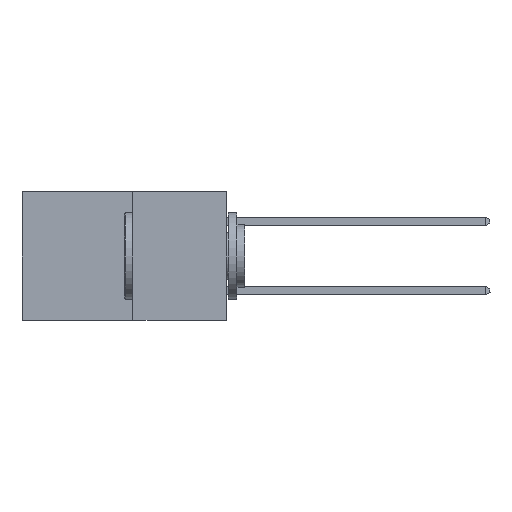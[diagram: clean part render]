
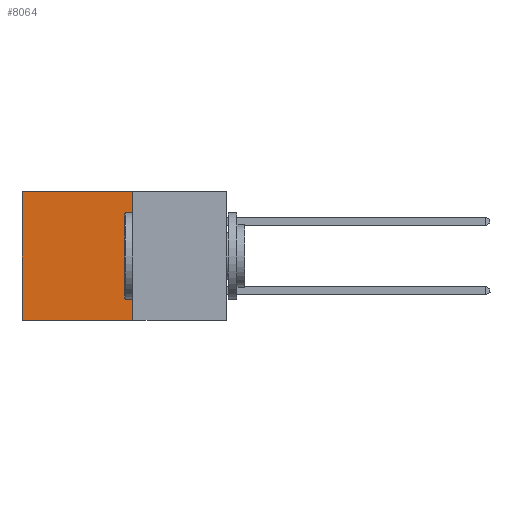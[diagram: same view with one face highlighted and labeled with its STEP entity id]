
A CAD part, left-side view. The second image highlights one B-rep face of the part: STEP entity #8064.
In plain terms, the highlighted planar face has unit normal (-1, 0, 0).
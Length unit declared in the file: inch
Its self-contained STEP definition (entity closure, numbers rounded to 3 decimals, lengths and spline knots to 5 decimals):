
#3552 = EDGE_CURVE ( 'NONE', #7562, #12265, #13279, .T. ) ;
#3914 = EDGE_CURVE ( 'NONE', #12431, #4497, #6377, .T. ) ;
#4263 = ORIENTED_EDGE ( 'NONE', *, *, #6254, .T. ) ;
#4317 = LINE ( 'NONE', #12335, #21337 ) ;
#4497 = VERTEX_POINT ( 'NONE', #16851 ) ;
#4714 = ORIENTED_EDGE ( 'NONE', *, *, #3552, .T. ) ;
#5039 = CARTESIAN_POINT ( 'NONE',  ( 0.277, 0.27, 0. ) ) ;
#5916 = LINE ( 'NONE', #16080, #13849 ) ;
#5930 = DIRECTION ( 'NONE',  ( 0., 0., -1. ) ) ;
#5969 = CARTESIAN_POINT ( 'NONE',  ( 0.277, 0.27, 0. ) ) ;
#6254 = EDGE_CURVE ( 'NONE', #12265, #4497, #4317, .T. ) ;
#6377 = LINE ( 'NONE', #14659, #6909 ) ;
#6710 = ORIENTED_EDGE ( 'NONE', *, *, #15152, .F. ) ;
#6909 = VECTOR ( 'NONE', #14686, 39.37008 ) ;
#7562 = VERTEX_POINT ( 'NONE', #5969 ) ;
#8064 = ADVANCED_FACE ( 'NONE', ( #17251 ), #18720, .F. ) ;
#9118 = EDGE_LOOP ( 'NONE', ( #4263, #14169, #6710, #4714 ) ) ;
#9193 = AXIS2_PLACEMENT_3D ( 'NONE', #18670, #18639, #18614 ) ;
#9762 = DIRECTION ( 'NONE',  ( 0., 1., 0. ) ) ;
#12130 = DIRECTION ( 'NONE',  ( 0., 0., -1. ) ) ;
#12265 = VERTEX_POINT ( 'NONE', #13928 ) ;
#12335 = CARTESIAN_POINT ( 'NONE',  ( 0.277, 0.59, -0.37 ) ) ;
#12431 = VERTEX_POINT ( 'NONE', #19424 ) ;
#13279 = LINE ( 'NONE', #5039, #21804 ) ;
#13849 = VECTOR ( 'NONE', #5930, 39.37008 ) ;
#13928 = CARTESIAN_POINT ( 'NONE',  ( 0.277, 0.59, 0. ) ) ;
#14169 = ORIENTED_EDGE ( 'NONE', *, *, #3914, .F. ) ;
#14659 = CARTESIAN_POINT ( 'NONE',  ( 0.277, 0.27, -0.37 ) ) ;
#14686 = DIRECTION ( 'NONE',  ( 0., 1., 0. ) ) ;
#15152 = EDGE_CURVE ( 'NONE', #7562, #12431, #5916, .T. ) ;
#16080 = CARTESIAN_POINT ( 'NONE',  ( 0.277, 0.27, -0.37 ) ) ;
#16851 = CARTESIAN_POINT ( 'NONE',  ( 0.277, 0.59, -0.37 ) ) ;
#17251 = FACE_OUTER_BOUND ( 'NONE', #9118, .T. ) ;
#18614 = DIRECTION ( 'NONE',  ( 0., 0., -1. ) ) ;
#18639 = DIRECTION ( 'NONE',  ( 1., 0., 0. ) ) ;
#18670 = CARTESIAN_POINT ( 'NONE',  ( 0.277, 0.27, -0.37 ) ) ;
#18720 = PLANE ( 'NONE',  #9193 ) ;
#19424 = CARTESIAN_POINT ( 'NONE',  ( 0.277, 0.27, -0.37 ) ) ;
#21337 = VECTOR ( 'NONE', #12130, 39.37008 ) ;
#21804 = VECTOR ( 'NONE', #9762, 39.37008 ) ;
